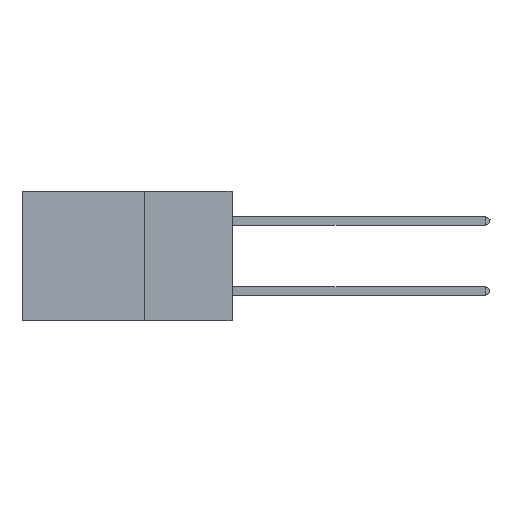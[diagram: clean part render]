
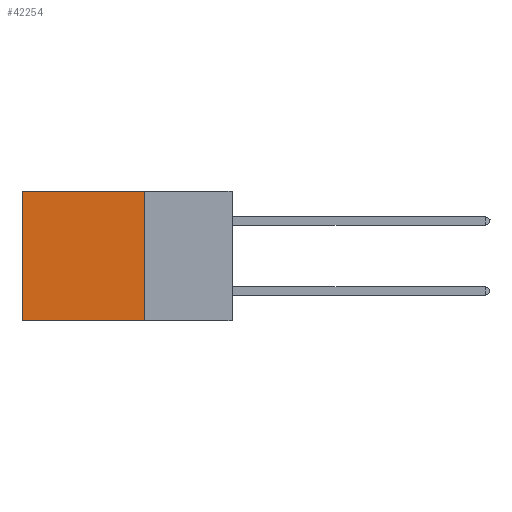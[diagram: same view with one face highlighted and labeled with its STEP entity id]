
A CAD part, left-side view. The second image highlights one B-rep face of the part: STEP entity #42254.
In plain terms, the highlighted planar face has unit normal (-1, 0, 0).
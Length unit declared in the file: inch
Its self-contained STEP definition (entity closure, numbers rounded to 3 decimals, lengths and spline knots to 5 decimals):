
#317 = PLANE ( 'NONE',  #1485 ) ;
#1485 = AXIS2_PLACEMENT_3D ( 'NONE', #24181, #6740, #37874 ) ;
#2923 = VECTOR ( 'NONE', #26629, 39.37008 ) ;
#6740 = DIRECTION ( 'NONE',  ( 1., 0., 0. ) ) ;
#7033 = CARTESIAN_POINT ( 'NONE',  ( 0.2875, 0.25, 0. ) ) ;
#7334 = EDGE_CURVE ( 'NONE', #8863, #38162, #9893, .T. ) ;
#8863 = VERTEX_POINT ( 'NONE', #31060 ) ;
#9893 = LINE ( 'NONE', #23371, #13857 ) ;
#10969 = ORIENTED_EDGE ( 'NONE', *, *, #30055, .T. ) ;
#13347 = ORIENTED_EDGE ( 'NONE', *, *, #18037, .F. ) ;
#13364 = LINE ( 'NONE', #30161, #28969 ) ;
#13857 = VECTOR ( 'NONE', #33303, 39.37008 ) ;
#17044 = VECTOR ( 'NONE', #20506, 39.37008 ) ;
#18037 = EDGE_CURVE ( 'NONE', #31475, #8863, #41046, .T. ) ;
#19783 = CARTESIAN_POINT ( 'NONE',  ( 0.2875, 0.25, 0. ) ) ;
#20506 = DIRECTION ( 'NONE',  ( 0., 0., -1. ) ) ;
#23371 = CARTESIAN_POINT ( 'NONE',  ( 0.2875, 0.25, -0.37 ) ) ;
#23811 = EDGE_LOOP ( 'NONE', ( #10969, #38784, #13347, #39119 ) ) ;
#24181 = CARTESIAN_POINT ( 'NONE',  ( 0.2875, 0.25, 0. ) ) ;
#26629 = DIRECTION ( 'NONE',  ( 0., 1., 0. ) ) ;
#28969 = VECTOR ( 'NONE', #31609, 39.37008 ) ;
#30055 = EDGE_CURVE ( 'NONE', #40864, #38162, #13364, .T. ) ;
#30161 = CARTESIAN_POINT ( 'NONE',  ( 0.2875, 0.6, 0. ) ) ;
#30375 = CARTESIAN_POINT ( 'NONE',  ( 0.2875, 0.6, 0. ) ) ;
#31060 = CARTESIAN_POINT ( 'NONE',  ( 0.2875, 0.25, -0.37 ) ) ;
#31475 = VERTEX_POINT ( 'NONE', #36286 ) ;
#31609 = DIRECTION ( 'NONE',  ( 0., 0., -1. ) ) ;
#33303 = DIRECTION ( 'NONE',  ( 0., 1., 0. ) ) ;
#34890 = CARTESIAN_POINT ( 'NONE',  ( 0.2875, 0.6, -0.37 ) ) ;
#36133 = LINE ( 'NONE', #19783, #2923 ) ;
#36286 = CARTESIAN_POINT ( 'NONE',  ( 0.2875, 0.25, 0. ) ) ;
#37874 = DIRECTION ( 'NONE',  ( 0., 0., -1. ) ) ;
#38162 = VERTEX_POINT ( 'NONE', #34890 ) ;
#38784 = ORIENTED_EDGE ( 'NONE', *, *, #7334, .F. ) ;
#39119 = ORIENTED_EDGE ( 'NONE', *, *, #40752, .T. ) ;
#40752 = EDGE_CURVE ( 'NONE', #31475, #40864, #36133, .T. ) ;
#40757 = FACE_OUTER_BOUND ( 'NONE', #23811, .T. ) ;
#40864 = VERTEX_POINT ( 'NONE', #30375 ) ;
#41046 = LINE ( 'NONE', #7033, #17044 ) ;
#42254 = ADVANCED_FACE ( 'NONE', ( #40757 ), #317, .F. ) ;
